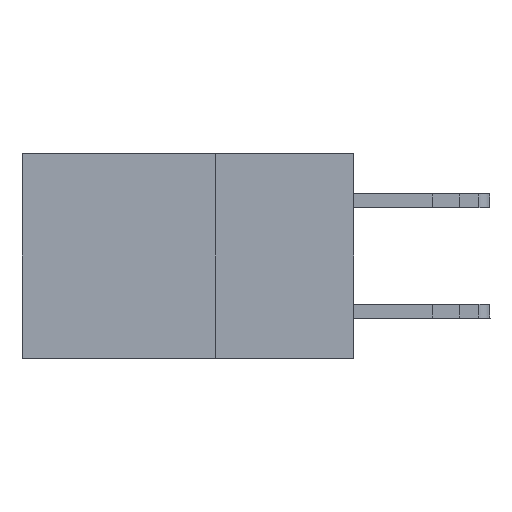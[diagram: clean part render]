
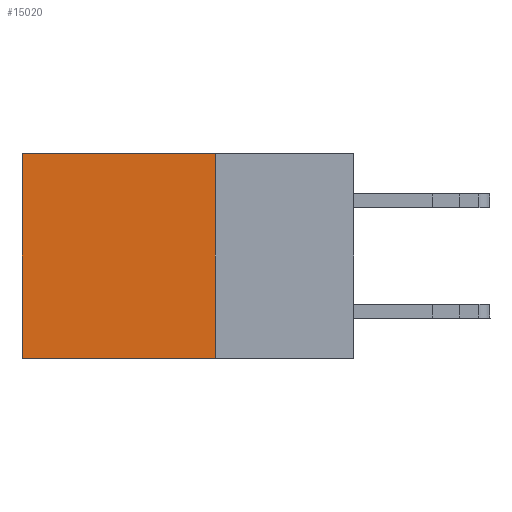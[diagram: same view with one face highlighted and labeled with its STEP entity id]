
A CAD part, left-side view. The second image highlights one B-rep face of the part: STEP entity #15020.
In plain terms, the highlighted planar face has unit normal (-1, 0, 0).
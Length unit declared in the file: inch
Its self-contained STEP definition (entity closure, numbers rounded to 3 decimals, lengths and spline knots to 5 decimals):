
#1228 = VERTEX_POINT ( 'NONE', #30644 ) ;
#1496 = DIRECTION ( 'NONE',  ( 0., 0., -1. ) ) ;
#1665 = LINE ( 'NONE', #28169, #26741 ) ;
#2177 = CARTESIAN_POINT ( 'NONE',  ( 0.2875, 0.25, -0.37 ) ) ;
#2327 = FACE_OUTER_BOUND ( 'NONE', #25098, .T. ) ;
#3436 = PLANE ( 'NONE',  #24212 ) ;
#6031 = DIRECTION ( 'NONE',  ( 0., 0., -1. ) ) ;
#6327 = CARTESIAN_POINT ( 'NONE',  ( 0.2875, 0.25, 0. ) ) ;
#6755 = VECTOR ( 'NONE', #6031, 39.37008 ) ;
#8425 = CARTESIAN_POINT ( 'NONE',  ( 0.2875, 0.6, 0. ) ) ;
#9213 = EDGE_CURVE ( 'NONE', #29257, #32942, #19966, .T. ) ;
#9670 = VECTOR ( 'NONE', #26531, 39.37008 ) ;
#10042 = DIRECTION ( 'NONE',  ( 0., 1., 0. ) ) ;
#10127 = CARTESIAN_POINT ( 'NONE',  ( 0.2875, 0.6, -0.37 ) ) ;
#10436 = ORIENTED_EDGE ( 'NONE', *, *, #9213, .F. ) ;
#11098 = VECTOR ( 'NONE', #17666, 39.37008 ) ;
#15020 = ADVANCED_FACE ( 'NONE', ( #2327 ), #3436, .F. ) ;
#16055 = ORIENTED_EDGE ( 'NONE', *, *, #23481, .T. ) ;
#16610 = CARTESIAN_POINT ( 'NONE',  ( 0.2875, 0.25, 0. ) ) ;
#17666 = DIRECTION ( 'NONE',  ( 0., 1., 0. ) ) ;
#19966 = LINE ( 'NONE', #2177, #11098 ) ;
#20536 = ORIENTED_EDGE ( 'NONE', *, *, #31272, .F. ) ;
#23239 = VERTEX_POINT ( 'NONE', #16610 ) ;
#23481 = EDGE_CURVE ( 'NONE', #23239, #1228, #1665, .T. ) ;
#24008 = ORIENTED_EDGE ( 'NONE', *, *, #26569, .T. ) ;
#24212 = AXIS2_PLACEMENT_3D ( 'NONE', #6327, #29722, #1496 ) ;
#25098 = EDGE_LOOP ( 'NONE', ( #24008, #10436, #20536, #16055 ) ) ;
#25829 = LINE ( 'NONE', #32007, #6755 ) ;
#26531 = DIRECTION ( 'NONE',  ( 0., 0., -1. ) ) ;
#26569 = EDGE_CURVE ( 'NONE', #1228, #32942, #33188, .T. ) ;
#26741 = VECTOR ( 'NONE', #10042, 39.37008 ) ;
#28169 = CARTESIAN_POINT ( 'NONE',  ( 0.2875, 0.25, 0. ) ) ;
#29257 = VERTEX_POINT ( 'NONE', #29544 ) ;
#29544 = CARTESIAN_POINT ( 'NONE',  ( 0.2875, 0.25, -0.37 ) ) ;
#29722 = DIRECTION ( 'NONE',  ( 1., 0., 0. ) ) ;
#30644 = CARTESIAN_POINT ( 'NONE',  ( 0.2875, 0.6, 0. ) ) ;
#31272 = EDGE_CURVE ( 'NONE', #23239, #29257, #25829, .T. ) ;
#32007 = CARTESIAN_POINT ( 'NONE',  ( 0.2875, 0.25, 0. ) ) ;
#32942 = VERTEX_POINT ( 'NONE', #10127 ) ;
#33188 = LINE ( 'NONE', #8425, #9670 ) ;
